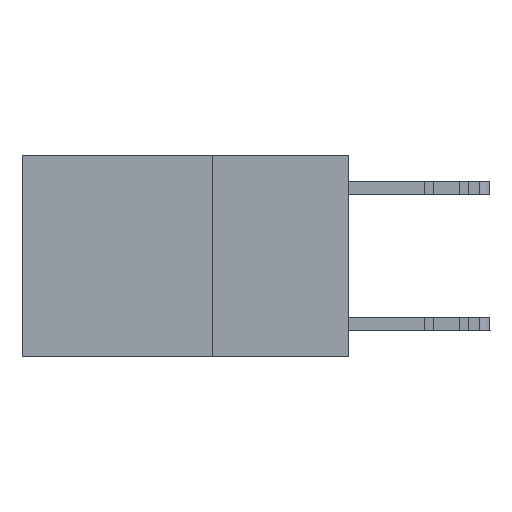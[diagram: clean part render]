
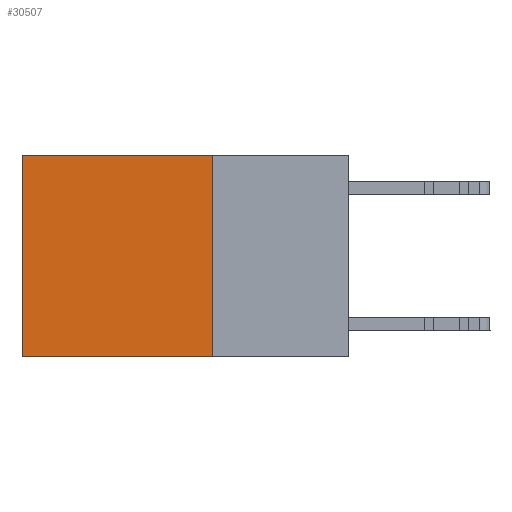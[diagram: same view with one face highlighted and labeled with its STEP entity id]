
A CAD part, left-side view. The second image highlights one B-rep face of the part: STEP entity #30507.
In plain terms, the highlighted planar face has unit normal (-1, 0, 0).
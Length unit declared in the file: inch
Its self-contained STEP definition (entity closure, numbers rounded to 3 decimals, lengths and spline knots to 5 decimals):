
#364 = LINE ( 'NONE', #30466, #5476 ) ;
#818 = CARTESIAN_POINT ( 'NONE',  ( 0.2625, 0.25, 0. ) ) ;
#1503 = VECTOR ( 'NONE', #17339, 39.37008 ) ;
#1675 = LINE ( 'NONE', #18577, #1503 ) ;
#2425 = ORIENTED_EDGE ( 'NONE', *, *, #29168, .T. ) ;
#3356 = CARTESIAN_POINT ( 'NONE',  ( 0.2625, 0.6, -0.37 ) ) ;
#3551 = LINE ( 'NONE', #818, #27988 ) ;
#3703 = CARTESIAN_POINT ( 'NONE',  ( 0.2625, 0.6, 0. ) ) ;
#4642 = CARTESIAN_POINT ( 'NONE',  ( 0.2625, 0.25, -0.37 ) ) ;
#4806 = PLANE ( 'NONE',  #21385 ) ;
#4938 = EDGE_LOOP ( 'NONE', ( #2425, #15319, #23932, #29102 ) ) ;
#5476 = VECTOR ( 'NONE', #14477, 39.37008 ) ;
#7254 = DIRECTION ( 'NONE',  ( 0., 0., -1. ) ) ;
#8818 = VERTEX_POINT ( 'NONE', #24649 ) ;
#9503 = CARTESIAN_POINT ( 'NONE',  ( 0.2625, 0.25, -0.37 ) ) ;
#10365 = FACE_OUTER_BOUND ( 'NONE', #4938, .T. ) ;
#11896 = DIRECTION ( 'NONE',  ( 0., 1., 0. ) ) ;
#14401 = CARTESIAN_POINT ( 'NONE',  ( 0.2625, 0.25, 0. ) ) ;
#14477 = DIRECTION ( 'NONE',  ( 0., 0., -1. ) ) ;
#15319 = ORIENTED_EDGE ( 'NONE', *, *, #16584, .F. ) ;
#15942 = EDGE_CURVE ( 'NONE', #8818, #19284, #1675, .T. ) ;
#16584 = EDGE_CURVE ( 'NONE', #19284, #24083, #24077, .T. ) ;
#17339 = DIRECTION ( 'NONE',  ( 0., 0., -1. ) ) ;
#18577 = CARTESIAN_POINT ( 'NONE',  ( 0.2625, 0.25, 0. ) ) ;
#19284 = VERTEX_POINT ( 'NONE', #4642 ) ;
#20118 = DIRECTION ( 'NONE',  ( 0., 1., 0. ) ) ;
#21385 = AXIS2_PLACEMENT_3D ( 'NONE', #14401, #21397, #7254 ) ;
#21397 = DIRECTION ( 'NONE',  ( 1., 0., 0. ) ) ;
#23491 = VERTEX_POINT ( 'NONE', #3703 ) ;
#23932 = ORIENTED_EDGE ( 'NONE', *, *, #15942, .F. ) ;
#24050 = VECTOR ( 'NONE', #11896, 39.37008 ) ;
#24077 = LINE ( 'NONE', #9503, #24050 ) ;
#24083 = VERTEX_POINT ( 'NONE', #3356 ) ;
#24649 = CARTESIAN_POINT ( 'NONE',  ( 0.2625, 0.25, 0. ) ) ;
#25310 = EDGE_CURVE ( 'NONE', #8818, #23491, #3551, .T. ) ;
#27988 = VECTOR ( 'NONE', #20118, 39.37008 ) ;
#29102 = ORIENTED_EDGE ( 'NONE', *, *, #25310, .T. ) ;
#29168 = EDGE_CURVE ( 'NONE', #23491, #24083, #364, .T. ) ;
#30466 = CARTESIAN_POINT ( 'NONE',  ( 0.2625, 0.6, 0. ) ) ;
#30507 = ADVANCED_FACE ( 'NONE', ( #10365 ), #4806, .F. ) ;
